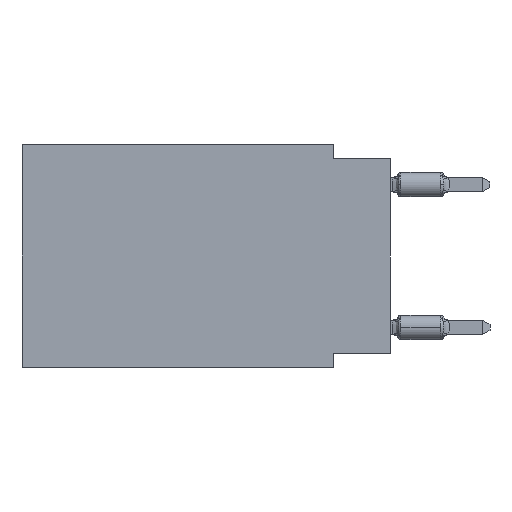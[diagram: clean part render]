
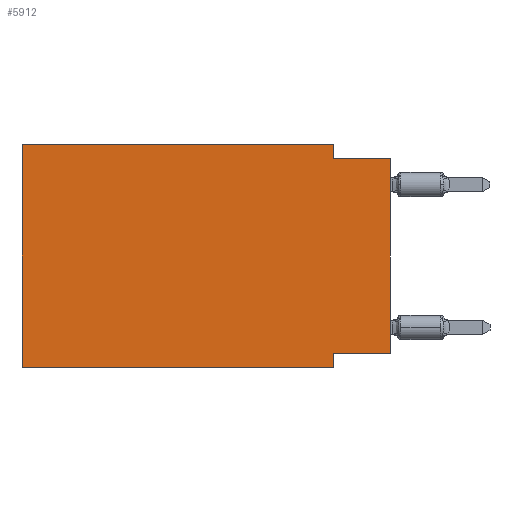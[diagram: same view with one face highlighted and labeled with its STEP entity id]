
A CAD part, left-side view. The second image highlights one B-rep face of the part: STEP entity #5912.
In plain terms, the highlighted planar face has unit normal (-1, 0, 0).
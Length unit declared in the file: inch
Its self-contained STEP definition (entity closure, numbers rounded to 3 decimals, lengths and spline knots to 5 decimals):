
#382 = CARTESIAN_POINT ( 'NONE',  ( 0., 0.1, -0.025 ) ) ;
#386 = VERTEX_POINT ( 'NONE', #19202 ) ;
#755 = CARTESIAN_POINT ( 'NONE',  ( 0., 0.645, -0.39 ) ) ;
#1006 = VERTEX_POINT ( 'NONE', #20072 ) ;
#1119 = VERTEX_POINT ( 'NONE', #382 ) ;
#1303 = LINE ( 'NONE', #15160, #2497 ) ;
#1332 = EDGE_CURVE ( 'NONE', #16068, #1006, #19348, .T. ) ;
#1798 = CARTESIAN_POINT ( 'NONE',  ( 0., 0.1, -0.365 ) ) ;
#1845 = CARTESIAN_POINT ( 'NONE',  ( 0., 0.645, -0.39 ) ) ;
#2497 = VECTOR ( 'NONE', #15058, 39.37008 ) ;
#3120 = ORIENTED_EDGE ( 'NONE', *, *, #1332, .F. ) ;
#3243 = VERTEX_POINT ( 'NONE', #9047 ) ;
#3417 = CARTESIAN_POINT ( 'NONE',  ( 0., 0., -0.365 ) ) ;
#4058 = CARTESIAN_POINT ( 'NONE',  ( 0., 0., -0.365 ) ) ;
#4286 = ORIENTED_EDGE ( 'NONE', *, *, #8317, .F. ) ;
#4410 = LINE ( 'NONE', #4720, #18832 ) ;
#4560 = LINE ( 'NONE', #6095, #13761 ) ;
#4720 = CARTESIAN_POINT ( 'NONE',  ( 0., 0.645, 0. ) ) ;
#5258 = VERTEX_POINT ( 'NONE', #755 ) ;
#5498 = LINE ( 'NONE', #4058, #12302 ) ;
#5546 = ORIENTED_EDGE ( 'NONE', *, *, #18005, .F. ) ;
#5598 = ORIENTED_EDGE ( 'NONE', *, *, #15266, .T. ) ;
#5912 = ADVANCED_FACE ( 'NONE', ( #14268 ), #12724, .F. ) ;
#6041 = VECTOR ( 'NONE', #10400, 39.37008 ) ;
#6095 = CARTESIAN_POINT ( 'NONE',  ( 0., 0.645, 0. ) ) ;
#7235 = AXIS2_PLACEMENT_3D ( 'NONE', #8184, #14365, #9686 ) ;
#7294 = EDGE_CURVE ( 'NONE', #5258, #15813, #4560, .T. ) ;
#7620 = VECTOR ( 'NONE', #19237, 39.37008 ) ;
#8059 = DIRECTION ( 'NONE',  ( 0., 0., 1. ) ) ;
#8184 = CARTESIAN_POINT ( 'NONE',  ( 0., 0.645, 0. ) ) ;
#8317 = EDGE_CURVE ( 'NONE', #3243, #1119, #8501, .T. ) ;
#8501 = LINE ( 'NONE', #19590, #6041 ) ;
#9047 = CARTESIAN_POINT ( 'NONE',  ( 0., 0.1, 0. ) ) ;
#9686 = DIRECTION ( 'NONE',  ( 0., 0., -1. ) ) ;
#10400 = DIRECTION ( 'NONE',  ( 0., 0., -1. ) ) ;
#10560 = DIRECTION ( 'NONE',  ( 0., 0., -1. ) ) ;
#10600 = ORIENTED_EDGE ( 'NONE', *, *, #12369, .T. ) ;
#10926 = DIRECTION ( 'NONE',  ( 0., -1., 0. ) ) ;
#12054 = EDGE_LOOP ( 'NONE', ( #10600, #13684, #4286, #5546, #13514, #5598, #3120, #14151 ) ) ;
#12302 = VECTOR ( 'NONE', #16484, 39.37008 ) ;
#12369 = EDGE_CURVE ( 'NONE', #12698, #386, #19339, .T. ) ;
#12698 = VERTEX_POINT ( 'NONE', #3417 ) ;
#12724 = PLANE ( 'NONE',  #7235 ) ;
#12993 = CARTESIAN_POINT ( 'NONE',  ( 0., 0., 0. ) ) ;
#13514 = ORIENTED_EDGE ( 'NONE', *, *, #7294, .F. ) ;
#13684 = ORIENTED_EDGE ( 'NONE', *, *, #17115, .F. ) ;
#13761 = VECTOR ( 'NONE', #8059, 39.37008 ) ;
#13868 = LINE ( 'NONE', #1845, #20028 ) ;
#14151 = ORIENTED_EDGE ( 'NONE', *, *, #19089, .F. ) ;
#14268 = FACE_OUTER_BOUND ( 'NONE', #12054, .T. ) ;
#14365 = DIRECTION ( 'NONE',  ( 1., 0., 0. ) ) ;
#15058 = DIRECTION ( 'NONE',  ( 0., -1., 0. ) ) ;
#15160 = CARTESIAN_POINT ( 'NONE',  ( 0., 0., -0.025 ) ) ;
#15266 = EDGE_CURVE ( 'NONE', #5258, #1006, #13868, .T. ) ;
#15813 = VERTEX_POINT ( 'NONE', #16090 ) ;
#16068 = VERTEX_POINT ( 'NONE', #1798 ) ;
#16090 = CARTESIAN_POINT ( 'NONE',  ( 0., 0.645, 0. ) ) ;
#16484 = DIRECTION ( 'NONE',  ( 0., 1., 0. ) ) ;
#17115 = EDGE_CURVE ( 'NONE', #1119, #386, #1303, .T. ) ;
#18005 = EDGE_CURVE ( 'NONE', #15813, #3243, #4410, .T. ) ;
#18531 = CARTESIAN_POINT ( 'NONE',  ( 0., 0.1, -0.39 ) ) ;
#18832 = VECTOR ( 'NONE', #10926, 39.37008 ) ;
#18834 = VECTOR ( 'NONE', #10560, 39.37008 ) ;
#19089 = EDGE_CURVE ( 'NONE', #12698, #16068, #5498, .T. ) ;
#19202 = CARTESIAN_POINT ( 'NONE',  ( 0., 0., -0.025 ) ) ;
#19237 = DIRECTION ( 'NONE',  ( 0., 0., 1. ) ) ;
#19339 = LINE ( 'NONE', #12993, #7620 ) ;
#19348 = LINE ( 'NONE', #18531, #18834 ) ;
#19590 = CARTESIAN_POINT ( 'NONE',  ( 0., 0.1, 0. ) ) ;
#20028 = VECTOR ( 'NONE', #20105, 39.37008 ) ;
#20072 = CARTESIAN_POINT ( 'NONE',  ( 0., 0.1, -0.39 ) ) ;
#20105 = DIRECTION ( 'NONE',  ( 0., -1., 0. ) ) ;
